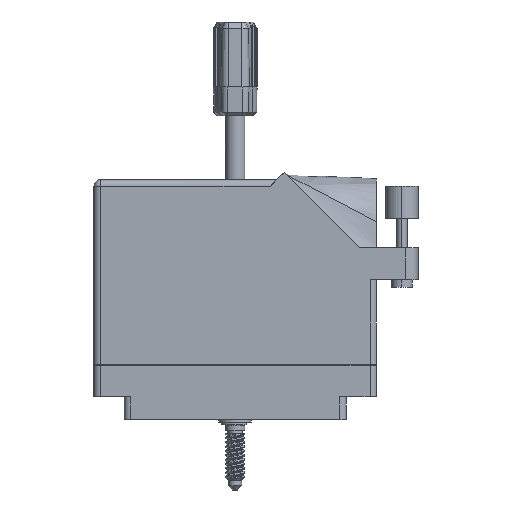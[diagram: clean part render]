
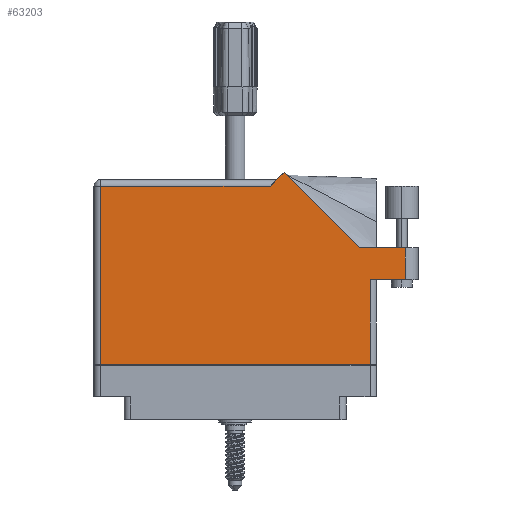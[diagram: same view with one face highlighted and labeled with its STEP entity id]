
A CAD part, front view. The second image highlights one B-rep face of the part: STEP entity #63203.
In plain terms, the highlighted face is planar.
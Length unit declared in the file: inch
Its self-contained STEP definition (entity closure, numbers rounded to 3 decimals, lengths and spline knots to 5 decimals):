
#1635 = EDGE_CURVE ( 'NONE', #53164, #48435, #40071, .T. ) ;
#1766 = ORIENTED_EDGE ( 'NONE', *, *, #1635, .T. ) ;
#1910 = DIRECTION ( 'NONE',  ( -1., 0., 0. ) ) ;
#2260 = EDGE_CURVE ( 'NONE', #66835, #53164, #59702, .T. ) ;
#6265 = DIRECTION ( 'NONE',  ( 0., -1., 0. ) ) ;
#6791 = CARTESIAN_POINT ( 'NONE',  ( -1.297, -0.1, 0.617 ) ) ;
#10021 = DIRECTION ( 'NONE',  ( -1., 0., 0. ) ) ;
#10473 = ORIENTED_EDGE ( 'NONE', *, *, #2260, .T. ) ;
#12029 = EDGE_CURVE ( 'NONE', #74961, #42696, #13281, .T. ) ;
#13281 = LINE ( 'NONE', #43025, #72128 ) ;
#14989 = CARTESIAN_POINT ( 'NONE',  ( 1.297, 0.715, 0.617 ) ) ;
#16345 = CARTESIAN_POINT ( 'NONE',  ( 1.759, 1.022, 0.617 ) ) ;
#16642 = ORIENTED_EDGE ( 'NONE', *, *, #35628, .T. ) ;
#22312 = LINE ( 'NONE', #6791, #25211 ) ;
#23741 = VECTOR ( 'NONE', #56073, 39.37008 ) ;
#25211 = VECTOR ( 'NONE', #6265, 39.37008 ) ;
#25530 = CARTESIAN_POINT ( 'NONE',  ( 0.399, 1.675, 0.617 ) ) ;
#26285 = DIRECTION ( 'NONE',  ( -0.707, -0.707, 0. ) ) ;
#26815 = DIRECTION ( 'NONE',  ( 0., 0., -1. ) ) ;
#26934 = FACE_OUTER_BOUND ( 'NONE', #79622, .T. ) ;
#27784 = CARTESIAN_POINT ( 'NONE',  ( 1.297, -0.1, 0.617 ) ) ;
#28027 = EDGE_CURVE ( 'NONE', #48435, #73482, #22312, .T. ) ;
#28907 = ORIENTED_EDGE ( 'NONE', *, *, #28027, .T. ) ;
#31081 = VECTOR ( 'NONE', #73054, 39.37008 ) ;
#31311 = CARTESIAN_POINT ( 'NONE',  ( -1.297, -0.1, 0.617 ) ) ;
#32029 = DIRECTION ( 'NONE',  ( 0., 1., 0. ) ) ;
#34675 = DIRECTION ( 'NONE',  ( 0., 1., 0. ) ) ;
#34719 = CARTESIAN_POINT ( 'NONE',  ( 1.634, 1.022, 0.617 ) ) ;
#35628 = EDGE_CURVE ( 'NONE', #42696, #78166, #77583, .T. ) ;
#36582 = DIRECTION ( 'NONE',  ( -1., 0., 0. ) ) ;
#36840 = DIRECTION ( 'NONE',  ( 1., 0., 0. ) ) ;
#37039 = EDGE_CURVE ( 'NONE', #78166, #50412, #74548, .T. ) ;
#37950 = LINE ( 'NONE', #72796, #31081 ) ;
#38549 = CARTESIAN_POINT ( 'NONE',  ( 0.46971, 1.74571, 0.617 ) ) ;
#40071 = LINE ( 'NONE', #62644, #52908 ) ;
#40084 = AXIS2_PLACEMENT_3D ( 'NONE', #76688, #26815, #1910 ) ;
#41897 = VECTOR ( 'NONE', #10021, 39.37008 ) ;
#42529 = ORIENTED_EDGE ( 'NONE', *, *, #56776, .T. ) ;
#42696 = VERTEX_POINT ( 'NONE', #14989 ) ;
#43025 = CARTESIAN_POINT ( 'NONE',  ( 1.297, 0.715, 0.617 ) ) ;
#43166 = VECTOR ( 'NONE', #34675, 39.37008 ) ;
#46532 = PLANE ( 'NONE',  #40084 ) ;
#46679 = CARTESIAN_POINT ( 'NONE',  ( -1.297, 1.613, 0.617 ) ) ;
#48435 = VERTEX_POINT ( 'NONE', #46679 ) ;
#48694 = VERTEX_POINT ( 'NONE', #63945 ) ;
#49010 = CARTESIAN_POINT ( 'NONE',  ( 0.337, 1.613, 0.617 ) ) ;
#50412 = VERTEX_POINT ( 'NONE', #34719 ) ;
#50779 = CARTESIAN_POINT ( 'NONE',  ( 1.359, 0.715, 0.617 ) ) ;
#52682 = ORIENTED_EDGE ( 'NONE', *, *, #56788, .T. ) ;
#52908 = VECTOR ( 'NONE', #36582, 39.37008 ) ;
#53164 = VERTEX_POINT ( 'NONE', #49010 ) ;
#55297 = ORIENTED_EDGE ( 'NONE', *, *, #37039, .T. ) ;
#56073 = DIRECTION ( 'NONE',  ( 1., 0., 0. ) ) ;
#56776 = EDGE_CURVE ( 'NONE', #50412, #48694, #73280, .T. ) ;
#56788 = EDGE_CURVE ( 'NONE', #48694, #66835, #37950, .T. ) ;
#59653 = VECTOR ( 'NONE', #36840, 39.37008 ) ;
#59702 = LINE ( 'NONE', #25530, #67588 ) ;
#60660 = EDGE_CURVE ( 'NONE', #73482, #74961, #76223, .T. ) ;
#62644 = CARTESIAN_POINT ( 'NONE',  ( -1.359, 1.613, 0.617 ) ) ;
#63203 = ADVANCED_FACE ( 'NONE', ( #26934 ), #46532, .F. ) ;
#63945 = CARTESIAN_POINT ( 'NONE',  ( 1.19342, 1.022, 0.617 ) ) ;
#65987 = CARTESIAN_POINT ( 'NONE',  ( 1.634, 1.022, 0.617 ) ) ;
#66835 = VERTEX_POINT ( 'NONE', #38549 ) ;
#67588 = VECTOR ( 'NONE', #26285, 39.37008 ) ;
#68655 = CARTESIAN_POINT ( 'NONE',  ( -1.359, -0.1, 0.617 ) ) ;
#70002 = CARTESIAN_POINT ( 'NONE',  ( 1.634, 0.715, 0.617 ) ) ;
#72128 = VECTOR ( 'NONE', #32029, 39.37008 ) ;
#72796 = CARTESIAN_POINT ( 'NONE',  ( 1.19342, 1.022, 0.617 ) ) ;
#73054 = DIRECTION ( 'NONE',  ( -0.707, 0.707, 0. ) ) ;
#73280 = LINE ( 'NONE', #16345, #41897 ) ;
#73482 = VERTEX_POINT ( 'NONE', #31311 ) ;
#74548 = LINE ( 'NONE', #65987, #43166 ) ;
#74743 = ORIENTED_EDGE ( 'NONE', *, *, #60660, .T. ) ;
#74961 = VERTEX_POINT ( 'NONE', #27784 ) ;
#76223 = LINE ( 'NONE', #68655, #59653 ) ;
#76688 = CARTESIAN_POINT ( 'NONE',  ( -1.359, 1.675, 0.617 ) ) ;
#77583 = LINE ( 'NONE', #50779, #23741 ) ;
#78166 = VERTEX_POINT ( 'NONE', #70002 ) ;
#79622 = EDGE_LOOP ( 'NONE', ( #16642, #55297, #42529, #52682, #10473, #1766, #28907, #74743, #81122 ) ) ;
#81122 = ORIENTED_EDGE ( 'NONE', *, *, #12029, .T. ) ;
